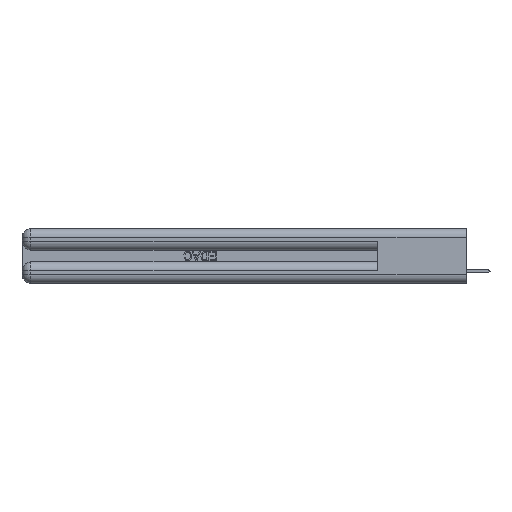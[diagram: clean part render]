
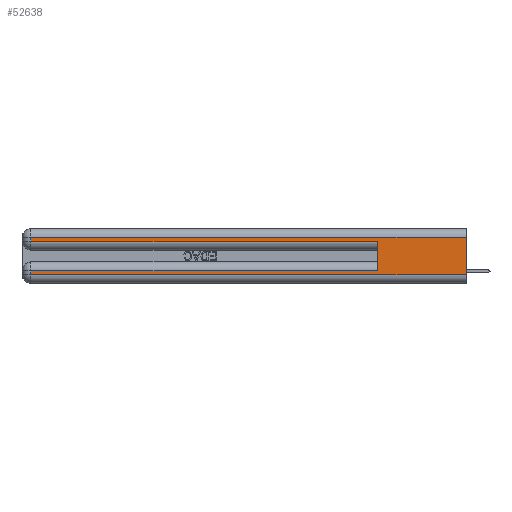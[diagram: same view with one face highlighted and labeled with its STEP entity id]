
A CAD part, left-side view. The second image highlights one B-rep face of the part: STEP entity #52638.
In plain terms, the highlighted planar face has unit normal (-1, 0, 0).
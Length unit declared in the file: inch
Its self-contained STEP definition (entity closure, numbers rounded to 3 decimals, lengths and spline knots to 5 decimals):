
#894 = VERTEX_POINT ( 'NONE', #3184 ) ;
#954 = LINE ( 'NONE', #20550, #44137 ) ;
#1109 = VECTOR ( 'NONE', #45762, 39.37008 ) ;
#1117 = VERTEX_POINT ( 'NONE', #20188 ) ;
#1467 = LINE ( 'NONE', #44229, #25724 ) ;
#3184 = CARTESIAN_POINT ( 'NONE',  ( 0., 2.94, 0.085 ) ) ;
#3352 = ORIENTED_EDGE ( 'NONE', *, *, #29256, .F. ) ;
#4760 = CARTESIAN_POINT ( 'NONE',  ( 0., 0., 0.285 ) ) ;
#5333 = VERTEX_POINT ( 'NONE', #8126 ) ;
#6945 = DIRECTION ( 'NONE',  ( 0., 1., 0. ) ) ;
#7299 = EDGE_CURVE ( 'NONE', #5333, #894, #47733, .T. ) ;
#7719 = DIRECTION ( 'NONE',  ( 0., -1., 0. ) ) ;
#8126 = CARTESIAN_POINT ( 'NONE',  ( 0., 0.6, 0.085 ) ) ;
#9226 = CARTESIAN_POINT ( 'NONE',  ( 0., 2.94, 0.285 ) ) ;
#10155 = LINE ( 'NONE', #29347, #42243 ) ;
#10759 = VERTEX_POINT ( 'NONE', #53654 ) ;
#13164 = VECTOR ( 'NONE', #7719, 39.37008 ) ;
#13271 = ORIENTED_EDGE ( 'NONE', *, *, #13949, .T. ) ;
#13949 = EDGE_CURVE ( 'NONE', #24670, #42671, #26910, .T. ) ;
#17422 = ORIENTED_EDGE ( 'NONE', *, *, #34051, .F. ) ;
#19194 = DIRECTION ( 'NONE',  ( 1., 0., 0. ) ) ;
#19566 = PLANE ( 'NONE',  #53053 ) ;
#20188 = CARTESIAN_POINT ( 'NONE',  ( 0., 2.94, 0.31 ) ) ;
#20550 = CARTESIAN_POINT ( 'NONE',  ( 0., 0., 0.37 ) ) ;
#21475 = VECTOR ( 'NONE', #44677, 39.37008 ) ;
#24670 = VERTEX_POINT ( 'NONE', #39472 ) ;
#25554 = VERTEX_POINT ( 'NONE', #48682 ) ;
#25724 = VECTOR ( 'NONE', #6945, 39.37008 ) ;
#26910 = LINE ( 'NONE', #53942, #13164 ) ;
#29256 = EDGE_CURVE ( 'NONE', #10759, #42671, #954, .T. ) ;
#29347 = CARTESIAN_POINT ( 'NONE',  ( 0., 2.94, 0.37 ) ) ;
#30389 = EDGE_LOOP ( 'NONE', ( #3352, #51878, #36862, #40061, #17422, #36425, #37000, #13271 ) ) ;
#30569 = VECTOR ( 'NONE', #34008, 39.37008 ) ;
#31130 = DIRECTION ( 'NONE',  ( 0., 1., 0. ) ) ;
#32939 = DIRECTION ( 'NONE',  ( 0., 0., -1. ) ) ;
#33188 = DIRECTION ( 'NONE',  ( 0., 0., -1. ) ) ;
#34008 = DIRECTION ( 'NONE',  ( 0., -1., 0. ) ) ;
#34051 = EDGE_CURVE ( 'NONE', #5333, #25554, #35778, .T. ) ;
#34485 = LINE ( 'NONE', #36058, #21475 ) ;
#34826 = CARTESIAN_POINT ( 'NONE',  ( 0., 0., 0.06 ) ) ;
#35778 = LINE ( 'NONE', #52217, #1109 ) ;
#36058 = CARTESIAN_POINT ( 'NONE',  ( 0., 2.94, 0.37 ) ) ;
#36425 = ORIENTED_EDGE ( 'NONE', *, *, #7299, .T. ) ;
#36862 = ORIENTED_EDGE ( 'NONE', *, *, #53826, .T. ) ;
#37000 = ORIENTED_EDGE ( 'NONE', *, *, #50464, .T. ) ;
#39472 = CARTESIAN_POINT ( 'NONE',  ( 0., 2.94, 0.06 ) ) ;
#40061 = ORIENTED_EDGE ( 'NONE', *, *, #44302, .T. ) ;
#42046 = FACE_OUTER_BOUND ( 'NONE', #30389, .T. ) ;
#42243 = VECTOR ( 'NONE', #33188, 39.37008 ) ;
#42671 = VERTEX_POINT ( 'NONE', #34826 ) ;
#43575 = CARTESIAN_POINT ( 'NONE',  ( 0., 0., 0.085 ) ) ;
#44137 = VECTOR ( 'NONE', #32939, 39.37008 ) ;
#44229 = CARTESIAN_POINT ( 'NONE',  ( 0., 0., 0.31 ) ) ;
#44302 = EDGE_CURVE ( 'NONE', #46485, #25554, #48289, .T. ) ;
#44417 = CARTESIAN_POINT ( 'NONE',  ( 0., 0., 0.37 ) ) ;
#44677 = DIRECTION ( 'NONE',  ( 0., 0., -1. ) ) ;
#45762 = DIRECTION ( 'NONE',  ( 0., 0., 1. ) ) ;
#46485 = VERTEX_POINT ( 'NONE', #9226 ) ;
#47733 = LINE ( 'NONE', #43575, #51037 ) ;
#48244 = DIRECTION ( 'NONE',  ( 0., 0., -1. ) ) ;
#48289 = LINE ( 'NONE', #4760, #30569 ) ;
#48682 = CARTESIAN_POINT ( 'NONE',  ( 0., 0.6, 0.285 ) ) ;
#50464 = EDGE_CURVE ( 'NONE', #894, #24670, #10155, .T. ) ;
#51037 = VECTOR ( 'NONE', #31130, 39.37008 ) ;
#51878 = ORIENTED_EDGE ( 'NONE', *, *, #52674, .T. ) ;
#52217 = CARTESIAN_POINT ( 'NONE',  ( 0., 0.6, 0.145 ) ) ;
#52638 = ADVANCED_FACE ( 'NONE', ( #42046 ), #19566, .F. ) ;
#52674 = EDGE_CURVE ( 'NONE', #10759, #1117, #1467, .T. ) ;
#53053 = AXIS2_PLACEMENT_3D ( 'NONE', #44417, #19194, #48244 ) ;
#53654 = CARTESIAN_POINT ( 'NONE',  ( 0., 0., 0.31 ) ) ;
#53826 = EDGE_CURVE ( 'NONE', #1117, #46485, #34485, .T. ) ;
#53942 = CARTESIAN_POINT ( 'NONE',  ( 0., 0., 0.06 ) ) ;
